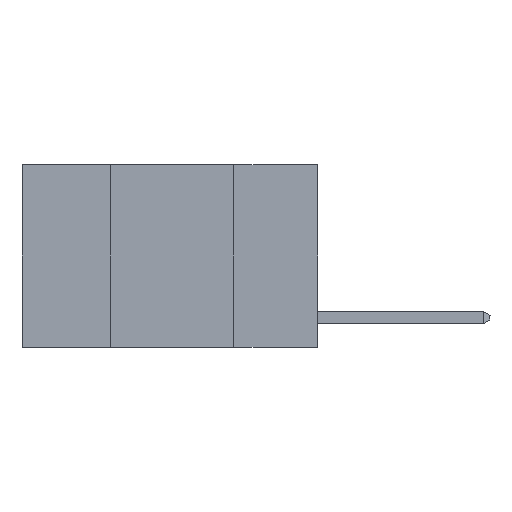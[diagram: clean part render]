
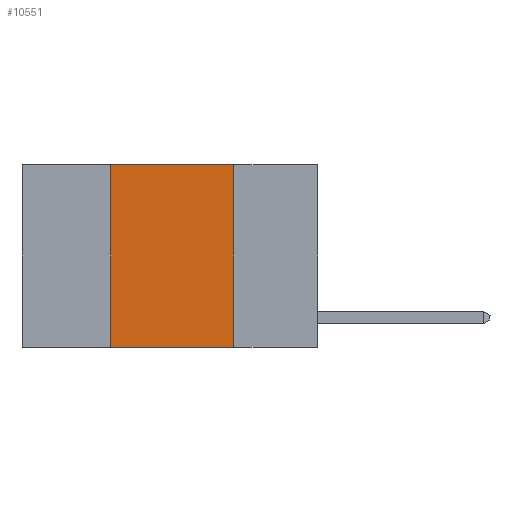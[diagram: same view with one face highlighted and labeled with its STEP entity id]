
A CAD part, left-side view. The second image highlights one B-rep face of the part: STEP entity #10551.
In plain terms, the highlighted planar face has unit normal (-1, 0, 0).
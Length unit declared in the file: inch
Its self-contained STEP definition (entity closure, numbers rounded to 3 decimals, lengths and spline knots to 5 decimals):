
#290 = LINE ( 'NONE', #7699, #2417 ) ;
#351 = VERTEX_POINT ( 'NONE', #4102 ) ;
#361 = DIRECTION ( 'NONE',  ( 1., 0., 0. ) ) ;
#901 = EDGE_LOOP ( 'NONE', ( #6551, #5257, #10062, #8564 ) ) ;
#2011 = VERTEX_POINT ( 'NONE', #3306 ) ;
#2116 = EDGE_CURVE ( 'NONE', #4809, #351, #10197, .T. ) ;
#2417 = VECTOR ( 'NONE', #9476, 39.37008 ) ;
#2428 = CARTESIAN_POINT ( 'NONE',  ( 0., 0.6, 0. ) ) ;
#2532 = LINE ( 'NONE', #2428, #3271 ) ;
#2882 = CARTESIAN_POINT ( 'NONE',  ( 0., 0.17, -0.37 ) ) ;
#3271 = VECTOR ( 'NONE', #10034, 39.37008 ) ;
#3306 = CARTESIAN_POINT ( 'NONE',  ( 0., 0.17, 0. ) ) ;
#4102 = CARTESIAN_POINT ( 'NONE',  ( 0., 0.42, 0. ) ) ;
#4221 = LINE ( 'NONE', #5132, #6207 ) ;
#4462 = DIRECTION ( 'NONE',  ( 0., 0., 1. ) ) ;
#4809 = VERTEX_POINT ( 'NONE', #5676 ) ;
#5053 = AXIS2_PLACEMENT_3D ( 'NONE', #8534, #361, #8421 ) ;
#5132 = CARTESIAN_POINT ( 'NONE',  ( 0., 0.17, 0. ) ) ;
#5248 = DIRECTION ( 'NONE',  ( 0., 0., -1. ) ) ;
#5257 = ORIENTED_EDGE ( 'NONE', *, *, #6094, .F. ) ;
#5312 = PLANE ( 'NONE',  #5053 ) ;
#5676 = CARTESIAN_POINT ( 'NONE',  ( 0., 0.42, -0.37 ) ) ;
#6094 = EDGE_CURVE ( 'NONE', #351, #2011, #2532, .T. ) ;
#6207 = VECTOR ( 'NONE', #5248, 39.37008 ) ;
#6551 = ORIENTED_EDGE ( 'NONE', *, *, #6666, .F. ) ;
#6666 = EDGE_CURVE ( 'NONE', #2011, #9837, #4221, .T. ) ;
#6993 = VECTOR ( 'NONE', #4462, 39.37008 ) ;
#7699 = CARTESIAN_POINT ( 'NONE',  ( 0., 0.6, -0.37 ) ) ;
#7971 = FACE_OUTER_BOUND ( 'NONE', #901, .T. ) ;
#8012 = EDGE_CURVE ( 'NONE', #4809, #9837, #290, .T. ) ;
#8421 = DIRECTION ( 'NONE',  ( 0., 0., -1. ) ) ;
#8534 = CARTESIAN_POINT ( 'NONE',  ( 0., 0.6, 0. ) ) ;
#8564 = ORIENTED_EDGE ( 'NONE', *, *, #8012, .T. ) ;
#9412 = CARTESIAN_POINT ( 'NONE',  ( 0., 0.42, 0. ) ) ;
#9476 = DIRECTION ( 'NONE',  ( 0., -1., 0. ) ) ;
#9837 = VERTEX_POINT ( 'NONE', #2882 ) ;
#10034 = DIRECTION ( 'NONE',  ( 0., -1., 0. ) ) ;
#10062 = ORIENTED_EDGE ( 'NONE', *, *, #2116, .F. ) ;
#10197 = LINE ( 'NONE', #9412, #6993 ) ;
#10551 = ADVANCED_FACE ( 'NONE', ( #7971 ), #5312, .F. ) ;
